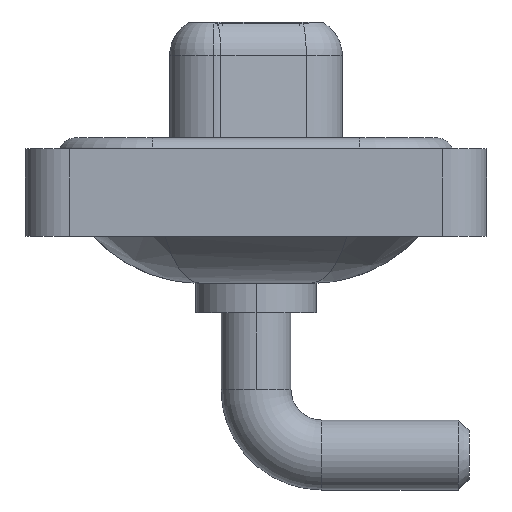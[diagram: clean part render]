
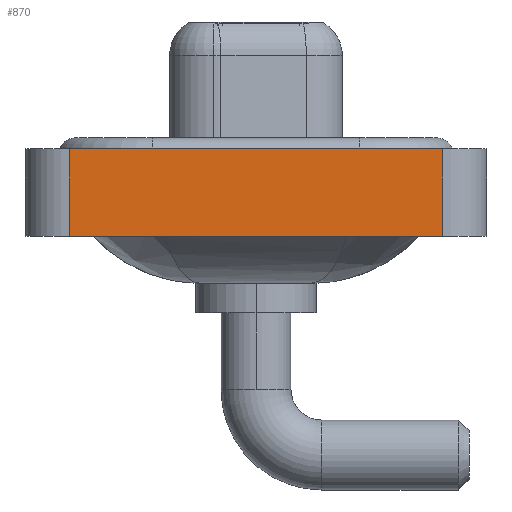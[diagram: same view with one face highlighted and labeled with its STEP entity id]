
A CAD part, left-side view. The second image highlights one B-rep face of the part: STEP entity #870.
In plain terms, the highlighted planar face has unit normal (-1, 0, 0).
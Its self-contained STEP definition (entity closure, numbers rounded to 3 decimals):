
#21 = ORIENTED_EDGE ( 'NONE', *, *, #13249, .T. ) ;
#534 = LINE ( 'NONE', #1806, #3610 ) ;
#660 = CARTESIAN_POINT ( 'NONE',  ( -7.25, 8.55, -3.6 ) ) ;
#870 = ADVANCED_FACE ( 'NONE', ( #13851 ), #2818, .T. ) ;
#1806 = CARTESIAN_POINT ( 'NONE',  ( -7.25, 8.55, -3.6 ) ) ;
#2208 = EDGE_LOOP ( 'NONE', ( #21, #13900, #4870, #10048 ) ) ;
#2222 = VERTEX_POINT ( 'NONE', #660 ) ;
#2818 = PLANE ( 'NONE',  #2819 ) ;
#2819 = AXIS2_PLACEMENT_3D ( 'NONE', #6478, #4090, #8922 ) ;
#3093 = CARTESIAN_POINT ( 'NONE',  ( -7.25, -8.55, -3.6 ) ) ;
#3610 = VECTOR ( 'NONE', #6643, 1000. ) ;
#3728 = CARTESIAN_POINT ( 'NONE',  ( -7.25, -8.55, 0.4 ) ) ;
#3753 = DIRECTION ( 'NONE',  ( 0., -1., 0. ) ) ;
#4090 = DIRECTION ( 'NONE',  ( -1., 0., 0. ) ) ;
#4870 = ORIENTED_EDGE ( 'NONE', *, *, #10905, .F. ) ;
#6352 = CARTESIAN_POINT ( 'NONE',  ( -7.25, -8.55, 0.4 ) ) ;
#6478 = CARTESIAN_POINT ( 'NONE',  ( -7.25, -8.55, -3.6 ) ) ;
#6643 = DIRECTION ( 'NONE',  ( 0., 0., 1. ) ) ;
#6695 = VECTOR ( 'NONE', #7831, 1000. ) ;
#7021 = CARTESIAN_POINT ( 'NONE',  ( -7.25, -8.55, -3.6 ) ) ;
#7831 = DIRECTION ( 'NONE',  ( 0., -1., 0. ) ) ;
#7948 = VERTEX_POINT ( 'NONE', #3728 ) ;
#8406 = CARTESIAN_POINT ( 'NONE',  ( -7.25, 8.55, 0.4 ) ) ;
#8922 = DIRECTION ( 'NONE',  ( 0., 0., 1. ) ) ;
#9898 = LINE ( 'NONE', #14675, #10260 ) ;
#10048 = ORIENTED_EDGE ( 'NONE', *, *, #14977, .T. ) ;
#10260 = VECTOR ( 'NONE', #11263, 1000. ) ;
#10905 = EDGE_CURVE ( 'NONE', #2222, #11832, #534, .T. ) ;
#11263 = DIRECTION ( 'NONE',  ( 0., 0., 1. ) ) ;
#11832 = VERTEX_POINT ( 'NONE', #8406 ) ;
#13249 = EDGE_CURVE ( 'NONE', #14216, #7948, #9898, .T. ) ;
#13332 = EDGE_CURVE ( 'NONE', #11832, #7948, #13576, .T. ) ;
#13576 = LINE ( 'NONE', #6352, #15033 ) ;
#13851 = FACE_OUTER_BOUND ( 'NONE', #2208, .T. ) ;
#13900 = ORIENTED_EDGE ( 'NONE', *, *, #13332, .F. ) ;
#14216 = VERTEX_POINT ( 'NONE', #7021 ) ;
#14675 = CARTESIAN_POINT ( 'NONE',  ( -7.25, -8.55, -3.6 ) ) ;
#14975 = LINE ( 'NONE', #3093, #6695 ) ;
#14977 = EDGE_CURVE ( 'NONE', #2222, #14216, #14975, .T. ) ;
#15033 = VECTOR ( 'NONE', #3753, 1000. ) ;
